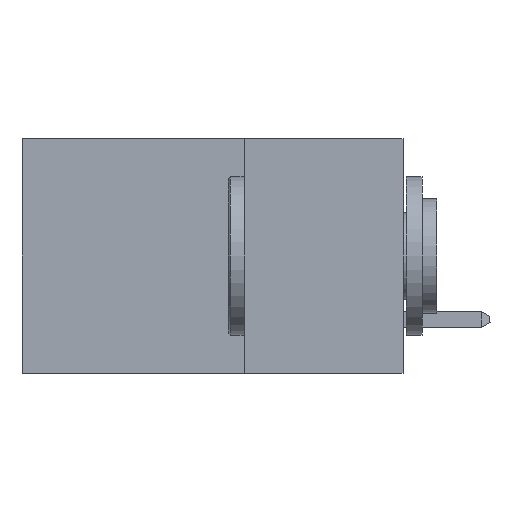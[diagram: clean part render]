
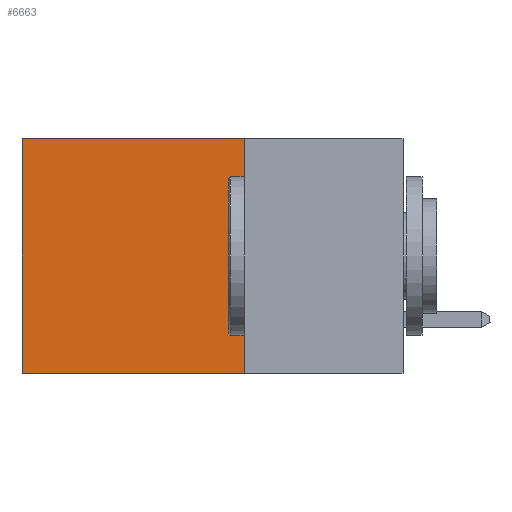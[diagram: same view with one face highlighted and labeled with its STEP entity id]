
A CAD part, left-side view. The second image highlights one B-rep face of the part: STEP entity #6663.
In plain terms, the highlighted planar face has unit normal (-1, 0, 0).
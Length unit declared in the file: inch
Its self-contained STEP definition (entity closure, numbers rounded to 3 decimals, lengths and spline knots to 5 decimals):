
#37 = EDGE_CURVE ( 'NONE', #8152, #5149, #7489, .T. ) ;
#124 = CARTESIAN_POINT ( 'NONE',  ( 0.2875, 0.25, -0.37 ) ) ;
#337 = DIRECTION ( 'NONE',  ( 0., 0., -1. ) ) ;
#528 = CARTESIAN_POINT ( 'NONE',  ( 0.2875, 0.25, 0. ) ) ;
#959 = ORIENTED_EDGE ( 'NONE', *, *, #37, .F. ) ;
#1435 = EDGE_CURVE ( 'NONE', #8152, #5202, #10169, .T. ) ;
#2001 = AXIS2_PLACEMENT_3D ( 'NONE', #528, #3617, #7606 ) ;
#2571 = VECTOR ( 'NONE', #7632, 39.37008 ) ;
#2873 = EDGE_CURVE ( 'NONE', #5149, #11150, #8254, .T. ) ;
#3036 = VECTOR ( 'NONE', #337, 39.37008 ) ;
#3152 = ORIENTED_EDGE ( 'NONE', *, *, #1435, .T. ) ;
#3165 = DIRECTION ( 'NONE',  ( 0., 1., 0. ) ) ;
#3540 = FACE_OUTER_BOUND ( 'NONE', #7368, .T. ) ;
#3617 = DIRECTION ( 'NONE',  ( 1., 0., 0. ) ) ;
#3879 = CARTESIAN_POINT ( 'NONE',  ( 0.2875, 0.6, -0.37 ) ) ;
#3903 = VECTOR ( 'NONE', #6949, 39.37008 ) ;
#4291 = CARTESIAN_POINT ( 'NONE',  ( 0.2875, 0.6, 0. ) ) ;
#5149 = VERTEX_POINT ( 'NONE', #124 ) ;
#5202 = VERTEX_POINT ( 'NONE', #4291 ) ;
#5663 = VECTOR ( 'NONE', #3165, 39.37008 ) ;
#5851 = PLANE ( 'NONE',  #2001 ) ;
#6663 = ADVANCED_FACE ( 'NONE', ( #3540 ), #5851, .F. ) ;
#6688 = CARTESIAN_POINT ( 'NONE',  ( 0.2875, 0.25, -0.37 ) ) ;
#6817 = ORIENTED_EDGE ( 'NONE', *, *, #2873, .F. ) ;
#6949 = DIRECTION ( 'NONE',  ( 0., 1., 0. ) ) ;
#7368 = EDGE_LOOP ( 'NONE', ( #9963, #6817, #959, #3152 ) ) ;
#7489 = LINE ( 'NONE', #7675, #2571 ) ;
#7606 = DIRECTION ( 'NONE',  ( 0., 0., -1. ) ) ;
#7632 = DIRECTION ( 'NONE',  ( 0., 0., -1. ) ) ;
#7675 = CARTESIAN_POINT ( 'NONE',  ( 0.2875, 0.25, 0. ) ) ;
#7706 = LINE ( 'NONE', #9969, #3036 ) ;
#7727 = CARTESIAN_POINT ( 'NONE',  ( 0.2875, 0.25, 0. ) ) ;
#8152 = VERTEX_POINT ( 'NONE', #7727 ) ;
#8254 = LINE ( 'NONE', #6688, #5663 ) ;
#9077 = EDGE_CURVE ( 'NONE', #5202, #11150, #7706, .T. ) ;
#9440 = CARTESIAN_POINT ( 'NONE',  ( 0.2875, 0.25, 0. ) ) ;
#9963 = ORIENTED_EDGE ( 'NONE', *, *, #9077, .T. ) ;
#9969 = CARTESIAN_POINT ( 'NONE',  ( 0.2875, 0.6, 0. ) ) ;
#10169 = LINE ( 'NONE', #9440, #3903 ) ;
#11150 = VERTEX_POINT ( 'NONE', #3879 ) ;
